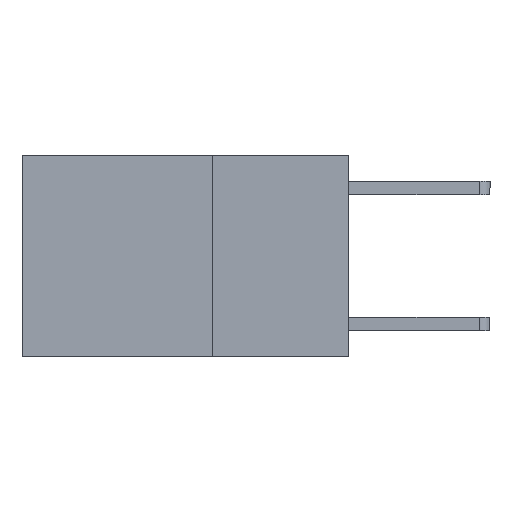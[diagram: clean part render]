
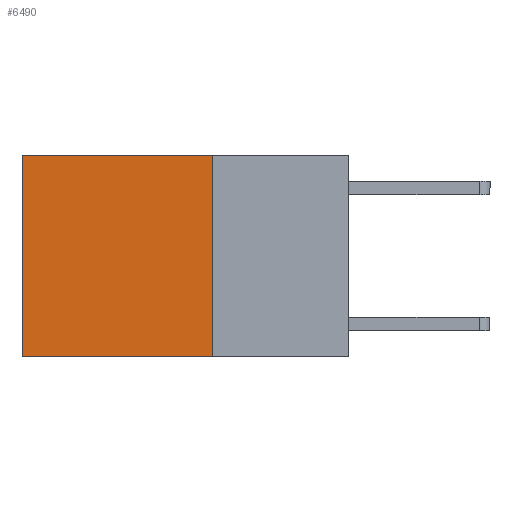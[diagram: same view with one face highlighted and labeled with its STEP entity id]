
A CAD part, left-side view. The second image highlights one B-rep face of the part: STEP entity #6490.
In plain terms, the highlighted planar face has unit normal (-1, 0, 0).
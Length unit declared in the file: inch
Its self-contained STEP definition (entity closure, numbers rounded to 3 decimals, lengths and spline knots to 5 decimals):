
#500 = VECTOR ( 'NONE', #5797, 39.37008 ) ;
#888 = DIRECTION ( 'NONE',  ( 1., 0., 0. ) ) ;
#1553 = PLANE ( 'NONE',  #2038 ) ;
#1812 = EDGE_LOOP ( 'NONE', ( #7601, #4368, #1908, #6973 ) ) ;
#1898 = CARTESIAN_POINT ( 'NONE',  ( 0.2625, 0.25, -0.37 ) ) ;
#1908 = ORIENTED_EDGE ( 'NONE', *, *, #4659, .F. ) ;
#2038 = AXIS2_PLACEMENT_3D ( 'NONE', #6928, #888, #3555 ) ;
#2083 = EDGE_CURVE ( 'NONE', #3223, #3196, #2566, .T. ) ;
#2566 = LINE ( 'NONE', #5237, #5615 ) ;
#2579 = DIRECTION ( 'NONE',  ( 0., 1., 0. ) ) ;
#2790 = EDGE_CURVE ( 'NONE', #4082, #3191, #4678, .T. ) ;
#3191 = VERTEX_POINT ( 'NONE', #7775 ) ;
#3196 = VERTEX_POINT ( 'NONE', #5158 ) ;
#3223 = VERTEX_POINT ( 'NONE', #7074 ) ;
#3555 = DIRECTION ( 'NONE',  ( 0., 0., -1. ) ) ;
#3662 = CARTESIAN_POINT ( 'NONE',  ( 0.2625, 0.6, 0. ) ) ;
#3919 = DIRECTION ( 'NONE',  ( 0., 1., 0. ) ) ;
#4082 = VERTEX_POINT ( 'NONE', #1898 ) ;
#4368 = ORIENTED_EDGE ( 'NONE', *, *, #2790, .F. ) ;
#4659 = EDGE_CURVE ( 'NONE', #3223, #4082, #5432, .T. ) ;
#4678 = LINE ( 'NONE', #5341, #4765 ) ;
#4765 = VECTOR ( 'NONE', #2579, 39.37008 ) ;
#5158 = CARTESIAN_POINT ( 'NONE',  ( 0.2625, 0.6, 0. ) ) ;
#5237 = CARTESIAN_POINT ( 'NONE',  ( 0.2625, 0.25, 0. ) ) ;
#5341 = CARTESIAN_POINT ( 'NONE',  ( 0.2625, 0.25, -0.37 ) ) ;
#5432 = LINE ( 'NONE', #6814, #6350 ) ;
#5553 = FACE_OUTER_BOUND ( 'NONE', #1812, .T. ) ;
#5615 = VECTOR ( 'NONE', #3919, 39.37008 ) ;
#5797 = DIRECTION ( 'NONE',  ( 0., 0., -1. ) ) ;
#6350 = VECTOR ( 'NONE', #8167, 39.37008 ) ;
#6464 = LINE ( 'NONE', #3662, #500 ) ;
#6490 = ADVANCED_FACE ( 'NONE', ( #5553 ), #1553, .F. ) ;
#6814 = CARTESIAN_POINT ( 'NONE',  ( 0.2625, 0.25, 0. ) ) ;
#6928 = CARTESIAN_POINT ( 'NONE',  ( 0.2625, 0.25, 0. ) ) ;
#6973 = ORIENTED_EDGE ( 'NONE', *, *, #2083, .T. ) ;
#7074 = CARTESIAN_POINT ( 'NONE',  ( 0.2625, 0.25, 0. ) ) ;
#7462 = EDGE_CURVE ( 'NONE', #3196, #3191, #6464, .T. ) ;
#7601 = ORIENTED_EDGE ( 'NONE', *, *, #7462, .T. ) ;
#7775 = CARTESIAN_POINT ( 'NONE',  ( 0.2625, 0.6, -0.37 ) ) ;
#8167 = DIRECTION ( 'NONE',  ( 0., 0., -1. ) ) ;
